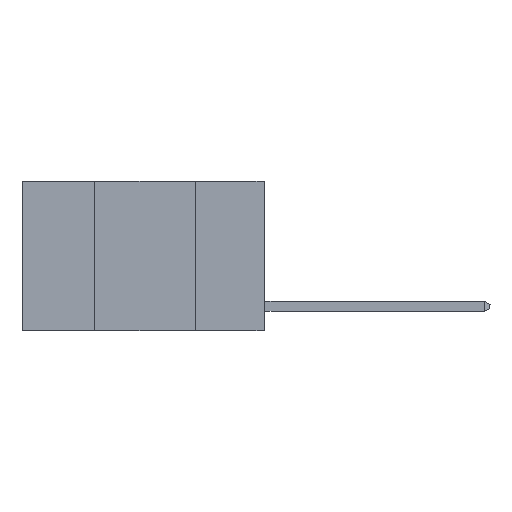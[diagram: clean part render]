
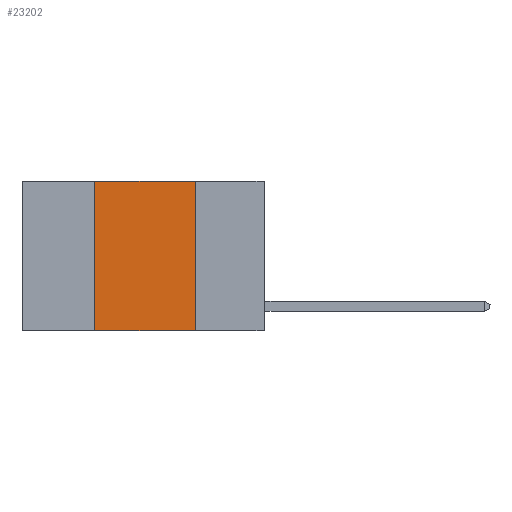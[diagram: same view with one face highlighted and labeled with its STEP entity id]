
A CAD part, left-side view. The second image highlights one B-rep face of the part: STEP entity #23202.
In plain terms, the highlighted planar face has unit normal (-1, 0, 0).
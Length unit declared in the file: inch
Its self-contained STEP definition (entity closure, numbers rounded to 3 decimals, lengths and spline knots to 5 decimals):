
#523 = ORIENTED_EDGE ( 'NONE', *, *, #15622, .F. ) ;
#2708 = DIRECTION ( 'NONE',  ( 1., 0., 0. ) ) ;
#2753 = VECTOR ( 'NONE', #24691, 39.37008 ) ;
#4307 = LINE ( 'NONE', #15183, #22510 ) ;
#5167 = VECTOR ( 'NONE', #28924, 39.37008 ) ;
#5831 = LINE ( 'NONE', #9963, #14483 ) ;
#8955 = CARTESIAN_POINT ( 'NONE',  ( 0., 0.17, -0.37 ) ) ;
#9748 = DIRECTION ( 'NONE',  ( 0., 0., -1. ) ) ;
#9963 = CARTESIAN_POINT ( 'NONE',  ( 0., 0.6, 0. ) ) ;
#11097 = CARTESIAN_POINT ( 'NONE',  ( 0., 0.17, 0. ) ) ;
#12747 = DIRECTION ( 'NONE',  ( 0., -1., 0. ) ) ;
#12775 = EDGE_CURVE ( 'NONE', #23703, #15337, #19955, .T. ) ;
#13322 = LINE ( 'NONE', #21889, #2753 ) ;
#13825 = CARTESIAN_POINT ( 'NONE',  ( 0., 0.42, 0. ) ) ;
#14483 = VECTOR ( 'NONE', #12747, 39.37008 ) ;
#15183 = CARTESIAN_POINT ( 'NONE',  ( 0., 0.6, -0.37 ) ) ;
#15337 = VERTEX_POINT ( 'NONE', #8955 ) ;
#15622 = EDGE_CURVE ( 'NONE', #26732, #23703, #5831, .T. ) ;
#15694 = EDGE_CURVE ( 'NONE', #20319, #26732, #13322, .T. ) ;
#16491 = AXIS2_PLACEMENT_3D ( 'NONE', #18738, #2708, #9748 ) ;
#17026 = ORIENTED_EDGE ( 'NONE', *, *, #15694, .F. ) ;
#17365 = CARTESIAN_POINT ( 'NONE',  ( 0., 0.42, -0.37 ) ) ;
#18738 = CARTESIAN_POINT ( 'NONE',  ( 0., 0.6, 0. ) ) ;
#19955 = LINE ( 'NONE', #11097, #5167 ) ;
#20319 = VERTEX_POINT ( 'NONE', #17365 ) ;
#20322 = EDGE_CURVE ( 'NONE', #20319, #15337, #4307, .T. ) ;
#20381 = FACE_OUTER_BOUND ( 'NONE', #25025, .T. ) ;
#21250 = ORIENTED_EDGE ( 'NONE', *, *, #12775, .F. ) ;
#21638 = ORIENTED_EDGE ( 'NONE', *, *, #20322, .T. ) ;
#21889 = CARTESIAN_POINT ( 'NONE',  ( 0., 0.42, 0. ) ) ;
#22510 = VECTOR ( 'NONE', #24167, 39.37008 ) ;
#23202 = ADVANCED_FACE ( 'NONE', ( #20381 ), #27145, .F. ) ;
#23703 = VERTEX_POINT ( 'NONE', #26975 ) ;
#24167 = DIRECTION ( 'NONE',  ( 0., -1., 0. ) ) ;
#24691 = DIRECTION ( 'NONE',  ( 0., 0., 1. ) ) ;
#25025 = EDGE_LOOP ( 'NONE', ( #21250, #523, #17026, #21638 ) ) ;
#26732 = VERTEX_POINT ( 'NONE', #13825 ) ;
#26975 = CARTESIAN_POINT ( 'NONE',  ( 0., 0.17, 0. ) ) ;
#27145 = PLANE ( 'NONE',  #16491 ) ;
#28924 = DIRECTION ( 'NONE',  ( 0., 0., -1. ) ) ;
